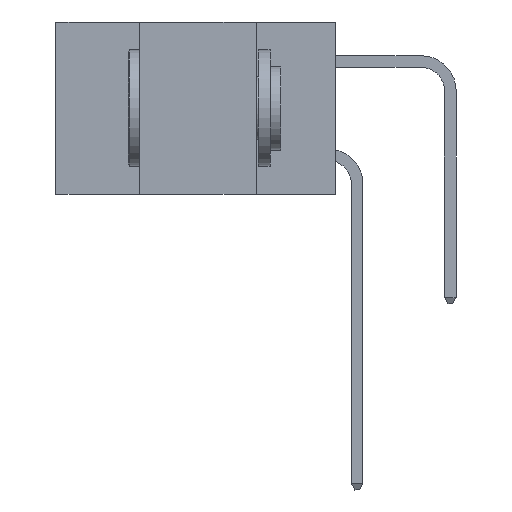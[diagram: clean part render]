
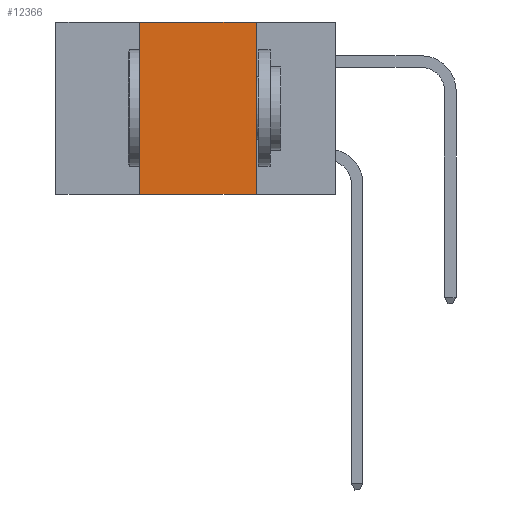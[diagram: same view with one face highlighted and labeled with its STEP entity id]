
A CAD part, left-side view. The second image highlights one B-rep face of the part: STEP entity #12366.
In plain terms, the highlighted planar face has unit normal (-1, 0, 0).
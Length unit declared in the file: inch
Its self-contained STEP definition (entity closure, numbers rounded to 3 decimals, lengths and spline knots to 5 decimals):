
#330 = EDGE_CURVE ( 'NONE', #13272, #11375, #1960, .T. ) ;
#656 = ORIENTED_EDGE ( 'NONE', *, *, #12704, .F. ) ;
#809 = LINE ( 'NONE', #11656, #3227 ) ;
#979 = AXIS2_PLACEMENT_3D ( 'NONE', #9302, #2382, #10513 ) ;
#1241 = EDGE_CURVE ( 'NONE', #14562, #11375, #14798, .T. ) ;
#1575 = VECTOR ( 'NONE', #8310, 39.37008 ) ;
#1960 = LINE ( 'NONE', #8119, #1575 ) ;
#2336 = PLANE ( 'NONE',  #979 ) ;
#2382 = DIRECTION ( 'NONE',  ( 1., 0., 0. ) ) ;
#3227 = VECTOR ( 'NONE', #3493, 39.37008 ) ;
#3493 = DIRECTION ( 'NONE',  ( 0., -1., 0. ) ) ;
#3991 = VECTOR ( 'NONE', #13512, 39.37008 ) ;
#5395 = VECTOR ( 'NONE', #14927, 39.37008 ) ;
#7640 = EDGE_CURVE ( 'NONE', #10079, #14562, #809, .T. ) ;
#7919 = CARTESIAN_POINT ( 'NONE',  ( 0., 0.42, 0. ) ) ;
#7980 = FACE_OUTER_BOUND ( 'NONE', #8842, .T. ) ;
#8119 = CARTESIAN_POINT ( 'NONE',  ( 0., 0.6, -0.37 ) ) ;
#8310 = DIRECTION ( 'NONE',  ( 0., -1., 0. ) ) ;
#8842 = EDGE_LOOP ( 'NONE', ( #14091, #12021, #656, #10929 ) ) ;
#9302 = CARTESIAN_POINT ( 'NONE',  ( 0., 0.6, 0. ) ) ;
#10079 = VERTEX_POINT ( 'NONE', #7919 ) ;
#10513 = DIRECTION ( 'NONE',  ( 0., 0., -1. ) ) ;
#10929 = ORIENTED_EDGE ( 'NONE', *, *, #330, .T. ) ;
#11182 = CARTESIAN_POINT ( 'NONE',  ( 0., 0.42, -0.37 ) ) ;
#11375 = VERTEX_POINT ( 'NONE', #12224 ) ;
#11656 = CARTESIAN_POINT ( 'NONE',  ( 0., 0.6, 0. ) ) ;
#12021 = ORIENTED_EDGE ( 'NONE', *, *, #7640, .F. ) ;
#12224 = CARTESIAN_POINT ( 'NONE',  ( 0., 0.17, -0.37 ) ) ;
#12293 = CARTESIAN_POINT ( 'NONE',  ( 0., 0.42, 0. ) ) ;
#12341 = CARTESIAN_POINT ( 'NONE',  ( 0., 0.17, 0. ) ) ;
#12366 = ADVANCED_FACE ( 'NONE', ( #7980 ), #2336, .F. ) ;
#12704 = EDGE_CURVE ( 'NONE', #13272, #10079, #13354, .T. ) ;
#13272 = VERTEX_POINT ( 'NONE', #11182 ) ;
#13354 = LINE ( 'NONE', #12293, #3991 ) ;
#13512 = DIRECTION ( 'NONE',  ( 0., 0., 1. ) ) ;
#14091 = ORIENTED_EDGE ( 'NONE', *, *, #1241, .F. ) ;
#14562 = VERTEX_POINT ( 'NONE', #12341 ) ;
#14798 = LINE ( 'NONE', #14892, #5395 ) ;
#14892 = CARTESIAN_POINT ( 'NONE',  ( 0., 0.17, 0. ) ) ;
#14927 = DIRECTION ( 'NONE',  ( 0., 0., -1. ) ) ;
